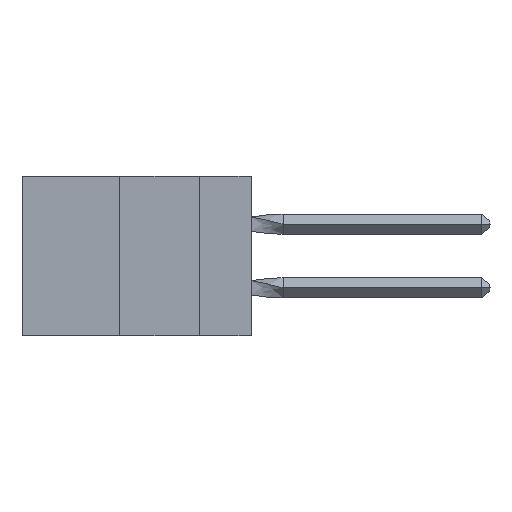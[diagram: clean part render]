
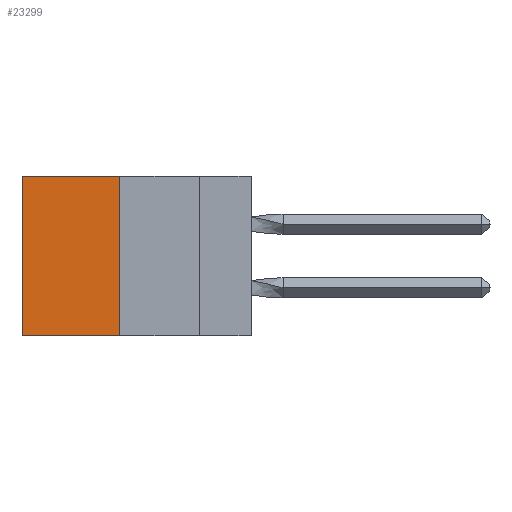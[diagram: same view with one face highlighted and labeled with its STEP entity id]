
A CAD part, left-side view. The second image highlights one B-rep face of the part: STEP entity #23299.
In plain terms, the highlighted planar face has unit normal (-1, 0, 0).
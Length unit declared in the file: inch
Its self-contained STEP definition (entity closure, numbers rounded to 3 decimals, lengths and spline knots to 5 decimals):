
#35 = DIRECTION ( 'NONE',  ( 0., 0., -1. ) ) ;
#291 = LINE ( 'NONE', #32983, #30376 ) ;
#445 = CARTESIAN_POINT ( 'NONE',  ( 0.305, 0.72, -0.5 ) ) ;
#3523 = ORIENTED_EDGE ( 'NONE', *, *, #19636, .T. ) ;
#6675 = DIRECTION ( 'NONE',  ( 0., 1., 0. ) ) ;
#8911 = DIRECTION ( 'NONE',  ( 0., 0., -1. ) ) ;
#10842 = EDGE_CURVE ( 'NONE', #31707, #25208, #291, .T. ) ;
#11003 = VECTOR ( 'NONE', #18798, 39.37008 ) ;
#11939 = DIRECTION ( 'NONE',  ( 0., 1., 0. ) ) ;
#12151 = VECTOR ( 'NONE', #11939, 39.37008 ) ;
#15683 = EDGE_CURVE ( 'NONE', #20564, #31707, #23554, .T. ) ;
#15780 = CARTESIAN_POINT ( 'NONE',  ( 0.305, 0.413, -0.5 ) ) ;
#17279 = EDGE_LOOP ( 'NONE', ( #3523, #24191, #34917, #21055 ) ) ;
#17998 = CARTESIAN_POINT ( 'NONE',  ( 0.305, 0.413, -0.5 ) ) ;
#18648 = FACE_OUTER_BOUND ( 'NONE', #17279, .T. ) ;
#18798 = DIRECTION ( 'NONE',  ( 0., 0., -1. ) ) ;
#19636 = EDGE_CURVE ( 'NONE', #37224, #25208, #25627, .T. ) ;
#20063 = LINE ( 'NONE', #35485, #12151 ) ;
#20129 = CARTESIAN_POINT ( 'NONE',  ( 0.305, 0.413, 0. ) ) ;
#20564 = VERTEX_POINT ( 'NONE', #20129 ) ;
#20862 = DIRECTION ( 'NONE',  ( 1., 0., 0. ) ) ;
#21055 = ORIENTED_EDGE ( 'NONE', *, *, #30888, .T. ) ;
#21177 = CARTESIAN_POINT ( 'NONE',  ( 0.305, 0.413, -0.5 ) ) ;
#22438 = VECTOR ( 'NONE', #35, 39.37008 ) ;
#23299 = ADVANCED_FACE ( 'NONE', ( #18648 ), #35718, .F. ) ;
#23554 = LINE ( 'NONE', #15780, #11003 ) ;
#24191 = ORIENTED_EDGE ( 'NONE', *, *, #10842, .F. ) ;
#25208 = VERTEX_POINT ( 'NONE', #445 ) ;
#25627 = LINE ( 'NONE', #29672, #22438 ) ;
#28201 = AXIS2_PLACEMENT_3D ( 'NONE', #17998, #20862, #8911 ) ;
#29534 = CARTESIAN_POINT ( 'NONE',  ( 0.305, 0.72, 0. ) ) ;
#29672 = CARTESIAN_POINT ( 'NONE',  ( 0.305, 0.72, -0.5 ) ) ;
#30376 = VECTOR ( 'NONE', #6675, 39.37008 ) ;
#30888 = EDGE_CURVE ( 'NONE', #20564, #37224, #20063, .T. ) ;
#31707 = VERTEX_POINT ( 'NONE', #21177 ) ;
#32983 = CARTESIAN_POINT ( 'NONE',  ( 0.305, 0.413, -0.5 ) ) ;
#34917 = ORIENTED_EDGE ( 'NONE', *, *, #15683, .F. ) ;
#35485 = CARTESIAN_POINT ( 'NONE',  ( 0.305, 0.413, 0. ) ) ;
#35718 = PLANE ( 'NONE',  #28201 ) ;
#37224 = VERTEX_POINT ( 'NONE', #29534 ) ;
